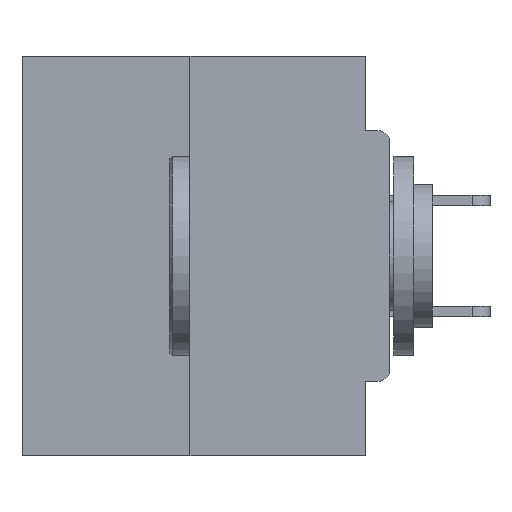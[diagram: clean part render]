
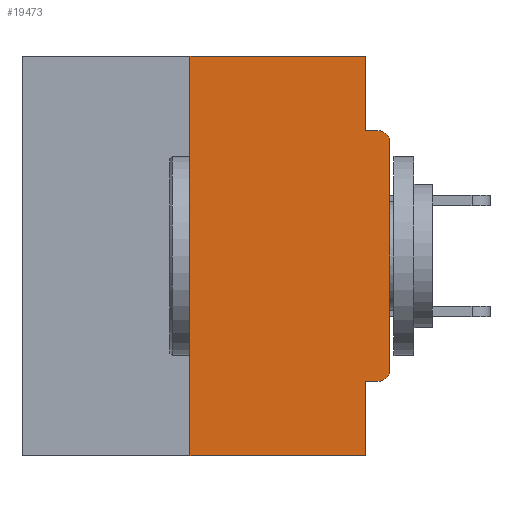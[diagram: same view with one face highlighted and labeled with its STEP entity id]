
A CAD part, left-side view. The second image highlights one B-rep face of the part: STEP entity #19473.
In plain terms, the highlighted planar face has unit normal (-1, 0, 0).
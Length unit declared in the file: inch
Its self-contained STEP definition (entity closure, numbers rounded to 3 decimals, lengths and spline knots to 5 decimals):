
#833 = DIRECTION ( 'NONE',  ( 0., -1., 0. ) ) ;
#1631 = DIRECTION ( 'NONE',  ( -1., 0., 0. ) ) ;
#2863 = CARTESIAN_POINT ( 'NONE',  ( 0., 0., -0.1085 ) ) ;
#3225 = EDGE_CURVE ( 'NONE', #18635, #9011, #11409, .T. ) ;
#3480 = LINE ( 'NONE', #6629, #14565 ) ;
#3508 = CARTESIAN_POINT ( 'NONE',  ( 0., 0.25, 0. ) ) ;
#3993 = CARTESIAN_POINT ( 'NONE',  ( 0., 0.015, -0.1085 ) ) ;
#4043 = EDGE_CURVE ( 'NONE', #4276, #4563, #24099, .T. ) ;
#4276 = VERTEX_POINT ( 'NONE', #32939 ) ;
#4336 = LINE ( 'NONE', #14609, #18591 ) ;
#4552 = DIRECTION ( 'NONE',  ( 0., -1., 0. ) ) ;
#4563 = VERTEX_POINT ( 'NONE', #23507 ) ;
#4844 = CARTESIAN_POINT ( 'NONE',  ( 0., 0.031, -0.0935 ) ) ;
#4956 = CARTESIAN_POINT ( 'NONE',  ( 0., 0.031, -0.5 ) ) ;
#5241 = PLANE ( 'NONE',  #18857 ) ;
#6371 = CARTESIAN_POINT ( 'NONE',  ( 0., 0.031, 0. ) ) ;
#6629 = CARTESIAN_POINT ( 'NONE',  ( 0., 0.25, 0. ) ) ;
#7673 = DIRECTION ( 'NONE',  ( 0., 0., -1. ) ) ;
#8025 = LINE ( 'NONE', #4956, #30722 ) ;
#8870 = DIRECTION ( 'NONE',  ( 0., 0., -1. ) ) ;
#9011 = VERTEX_POINT ( 'NONE', #6371 ) ;
#9435 = ORIENTED_EDGE ( 'NONE', *, *, #17200, .T. ) ;
#9574 = EDGE_CURVE ( 'NONE', #17178, #26366, #22568, .T. ) ;
#9973 = FACE_OUTER_BOUND ( 'NONE', #20168, .T. ) ;
#10110 = CARTESIAN_POINT ( 'NONE',  ( 0., 0.46, 0. ) ) ;
#10336 = ORIENTED_EDGE ( 'NONE', *, *, #3225, .F. ) ;
#10389 = ORIENTED_EDGE ( 'NONE', *, *, #9574, .T. ) ;
#11409 = LINE ( 'NONE', #10110, #16547 ) ;
#12444 = VECTOR ( 'NONE', #8870, 39.37008 ) ;
#12518 = ORIENTED_EDGE ( 'NONE', *, *, #32731, .F. ) ;
#12577 = DIRECTION ( 'NONE',  ( 0., 0., -1. ) ) ;
#12756 = DIRECTION ( 'NONE',  ( 1., 0., 0. ) ) ;
#14315 = AXIS2_PLACEMENT_3D ( 'NONE', #3993, #1631, #21827 ) ;
#14565 = VECTOR ( 'NONE', #24470, 39.37008 ) ;
#14609 = CARTESIAN_POINT ( 'NONE',  ( 0., 0., -0.4065 ) ) ;
#14682 = ORIENTED_EDGE ( 'NONE', *, *, #26483, .F. ) ;
#14757 = ORIENTED_EDGE ( 'NONE', *, *, #25952, .T. ) ;
#15024 = DIRECTION ( 'NONE',  ( -1., 0., 0. ) ) ;
#15926 = ORIENTED_EDGE ( 'NONE', *, *, #4043, .T. ) ;
#16403 = LINE ( 'NONE', #29418, #12444 ) ;
#16547 = VECTOR ( 'NONE', #4552, 39.37008 ) ;
#17178 = VERTEX_POINT ( 'NONE', #2863 ) ;
#17200 = EDGE_CURVE ( 'NONE', #19437, #17178, #28038, .T. ) ;
#18397 = CARTESIAN_POINT ( 'NONE',  ( 0., 0.46, -0.5 ) ) ;
#18591 = VECTOR ( 'NONE', #19812, 39.37008 ) ;
#18635 = VERTEX_POINT ( 'NONE', #3508 ) ;
#18857 = AXIS2_PLACEMENT_3D ( 'NONE', #22878, #12756, #7673 ) ;
#18934 = CARTESIAN_POINT ( 'NONE',  ( 0., 0.015, -0.4065 ) ) ;
#19437 = VERTEX_POINT ( 'NONE', #30595 ) ;
#19473 = ADVANCED_FACE ( 'NONE', ( #9973 ), #5241, .F. ) ;
#19812 = DIRECTION ( 'NONE',  ( 0., 1., 0. ) ) ;
#20107 = CARTESIAN_POINT ( 'NONE',  ( 0., 0.015, -0.3915 ) ) ;
#20168 = EDGE_LOOP ( 'NONE', ( #10336, #23581, #15926, #21266, #12518, #14757, #9435, #10389, #24040, #14682 ) ) ;
#21080 = DIRECTION ( 'NONE',  ( 0., -1., 0. ) ) ;
#21220 = CARTESIAN_POINT ( 'NONE',  ( 0., 0., -0.0935 ) ) ;
#21266 = ORIENTED_EDGE ( 'NONE', *, *, #27969, .F. ) ;
#21559 = EDGE_CURVE ( 'NONE', #4276, #18635, #3480, .T. ) ;
#21827 = DIRECTION ( 'NONE',  ( 0., 0., -1. ) ) ;
#22031 = VECTOR ( 'NONE', #28211, 39.37008 ) ;
#22351 = LINE ( 'NONE', #21220, #23528 ) ;
#22568 = CIRCLE ( 'NONE', #14315, 0.015 ) ;
#22878 = CARTESIAN_POINT ( 'NONE',  ( 0., 0.46, 0. ) ) ;
#23404 = VERTEX_POINT ( 'NONE', #18934 ) ;
#23507 = CARTESIAN_POINT ( 'NONE',  ( 0., 0.031, -0.5 ) ) ;
#23528 = VECTOR ( 'NONE', #833, 39.37008 ) ;
#23581 = ORIENTED_EDGE ( 'NONE', *, *, #21559, .F. ) ;
#23759 = EDGE_CURVE ( 'NONE', #30519, #26366, #22351, .T. ) ;
#24040 = ORIENTED_EDGE ( 'NONE', *, *, #23759, .F. ) ;
#24099 = LINE ( 'NONE', #18397, #26105 ) ;
#24470 = DIRECTION ( 'NONE',  ( 0., 0., 1. ) ) ;
#25603 = AXIS2_PLACEMENT_3D ( 'NONE', #20107, #15024, #12577 ) ;
#25952 = EDGE_CURVE ( 'NONE', #23404, #19437, #32360, .T. ) ;
#26105 = VECTOR ( 'NONE', #21080, 39.37008 ) ;
#26366 = VERTEX_POINT ( 'NONE', #30134 ) ;
#26483 = EDGE_CURVE ( 'NONE', #9011, #30519, #16403, .T. ) ;
#26747 = CARTESIAN_POINT ( 'NONE',  ( 0., 0.031, -0.4065 ) ) ;
#27886 = CARTESIAN_POINT ( 'NONE',  ( 0., 0., 0. ) ) ;
#27969 = EDGE_CURVE ( 'NONE', #30403, #4563, #8025, .T. ) ;
#28038 = LINE ( 'NONE', #27886, #22031 ) ;
#28211 = DIRECTION ( 'NONE',  ( 0., 0., 1. ) ) ;
#29418 = CARTESIAN_POINT ( 'NONE',  ( 0., 0.031, 0. ) ) ;
#30134 = CARTESIAN_POINT ( 'NONE',  ( 0., 0.015, -0.0935 ) ) ;
#30198 = DIRECTION ( 'NONE',  ( 0., 0., -1. ) ) ;
#30403 = VERTEX_POINT ( 'NONE', #26747 ) ;
#30519 = VERTEX_POINT ( 'NONE', #4844 ) ;
#30595 = CARTESIAN_POINT ( 'NONE',  ( 0., 0., -0.3915 ) ) ;
#30722 = VECTOR ( 'NONE', #30198, 39.37008 ) ;
#32360 = CIRCLE ( 'NONE', #25603, 0.015 ) ;
#32731 = EDGE_CURVE ( 'NONE', #23404, #30403, #4336, .T. ) ;
#32939 = CARTESIAN_POINT ( 'NONE',  ( 0., 0.25, -0.5 ) ) ;
